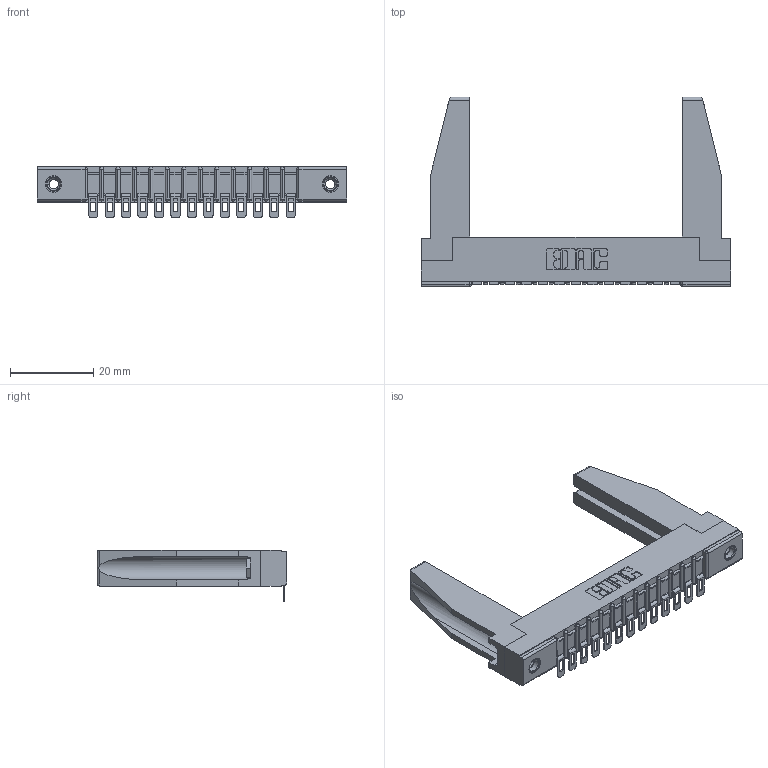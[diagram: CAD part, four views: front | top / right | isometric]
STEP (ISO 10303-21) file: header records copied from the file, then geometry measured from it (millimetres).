
FILE_DESCRIPTION (( 'STEP AP203' ), '1' );
FILE_NAME ('357-013-454-178.STEP', '2020-09-30T14:45:30', ( '' ), ( '' ), 'SwSTEP 2.0', 'SolidWorks 2020', '' );
FILE_SCHEMA (( 'CONFIG_CONTROL_DESIGN' ));
Length unit declared in the file: inch
Products named in the file (5): 357-013-454-178; 307-220-078; 345-250-001_345-250-001-102; 307-290-002_554; 307 Part_.156 Dia Mounting Holes
Assembly tree (18 placements, depth 2):
  357-013-454-178
    307 Part_.156 Dia Mounting Holes
    307-290-002_554  x13
    307-220-078  x2
    345-250-001_345-250-001-102  x2
Bounding box: 74.52 x 45.72 x 12.52 mm (x, y, z)
Volume: 8913.2 mm3; surface area: 12322.3 mm2
Topology: 18 solids, 18 shells, 1315 faces, 3942 edges, 2580 vertices
Faces by surface type: plane 752, cylinder 519, sphere 28, cone 12, torus 4
Entity records: 18124 total; most frequent: CARTESIAN_POINT 3052, ORIENTED_EDGE 2998, DIRECTION 2941, EDGE_CURVE 1499, VECTOR 1131, LINE 1131, VERTEX_POINT 974, AXIS2_PLACEMENT_3D 905
